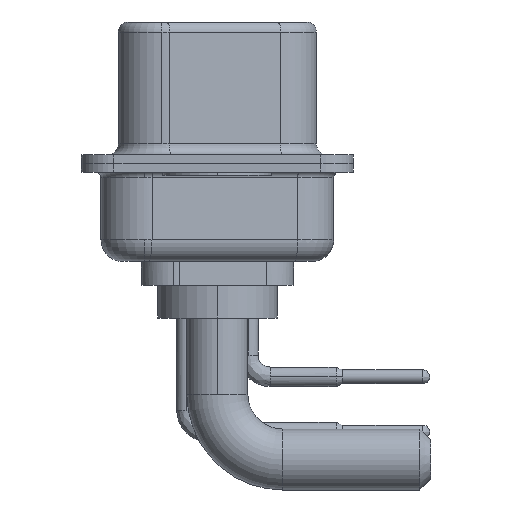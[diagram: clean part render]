
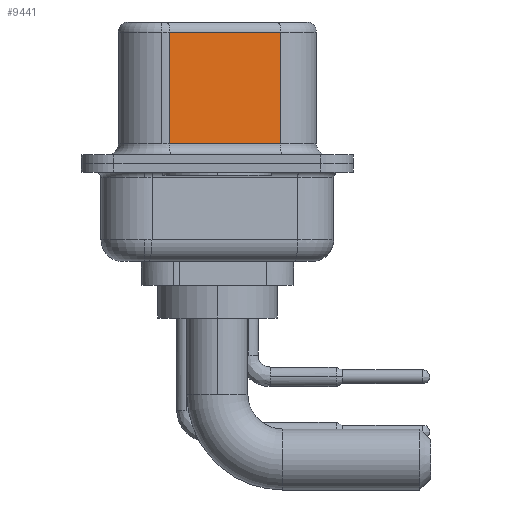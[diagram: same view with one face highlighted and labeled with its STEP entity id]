
A CAD part, left-side view. The second image highlights one B-rep face of the part: STEP entity #9441.
In plain terms, the highlighted planar face has unit normal (-0.985, -0.174, 0).
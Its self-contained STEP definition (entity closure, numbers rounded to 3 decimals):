
#51 = VERTEX_POINT ( 'NONE', #4802 ) ;
#521 = EDGE_CURVE ( 'NONE', #51, #2622, #3120, .T. ) ;
#622 = VECTOR ( 'NONE', #1052, 1000. ) ;
#881 = VECTOR ( 'NONE', #7619, 1000. ) ;
#1052 = DIRECTION ( 'NONE',  ( 0., 0., -1. ) ) ;
#1606 = DIRECTION ( 'NONE',  ( 0., 0., -1. ) ) ;
#1619 = FACE_OUTER_BOUND ( 'NONE', #7997, .T. ) ;
#2414 = CARTESIAN_POINT ( 'NONE',  ( 4.58, -2.897, 0.9 ) ) ;
#2622 = VERTEX_POINT ( 'NONE', #2414 ) ;
#3120 = LINE ( 'NONE', #12028, #15131 ) ;
#4802 = CARTESIAN_POINT ( 'NONE',  ( 3.68, 2.203, 0.9 ) ) ;
#5109 = PLANE ( 'NONE',  #15788 ) ;
#6396 = EDGE_CURVE ( 'NONE', #9933, #2622, #8262, .T. ) ;
#7048 = CARTESIAN_POINT ( 'NONE',  ( 4.58, -2.897, 6.02 ) ) ;
#7619 = DIRECTION ( 'NONE',  ( -0.174, 0.985, 0. ) ) ;
#7997 = EDGE_LOOP ( 'NONE', ( #20481, #19093, #16789, #13719 ) ) ;
#8262 = LINE ( 'NONE', #20416, #622 ) ;
#8454 = CARTESIAN_POINT ( 'NONE',  ( 3.68, 2.203, 6.52 ) ) ;
#8680 = LINE ( 'NONE', #8454, #10190 ) ;
#9441 = ADVANCED_FACE ( 'NONE', ( #1619 ), #5109, .F. ) ;
#9933 = VERTEX_POINT ( 'NONE', #7048 ) ;
#10190 = VECTOR ( 'NONE', #1606, 1000. ) ;
#10282 = DIRECTION ( 'NONE',  ( 0.174, -0.985, 0. ) ) ;
#12028 = CARTESIAN_POINT ( 'NONE',  ( 4.58, -2.897, 0.9 ) ) ;
#12046 = CARTESIAN_POINT ( 'NONE',  ( 4.58, -2.897, 6.52 ) ) ;
#13192 = EDGE_CURVE ( 'NONE', #9933, #13405, #18045, .T. ) ;
#13405 = VERTEX_POINT ( 'NONE', #13735 ) ;
#13719 = ORIENTED_EDGE ( 'NONE', *, *, #521, .T. ) ;
#13735 = CARTESIAN_POINT ( 'NONE',  ( 3.68, 2.203, 6.02 ) ) ;
#13774 = DIRECTION ( 'NONE',  ( -0.174, 0.985, 0. ) ) ;
#14992 = CARTESIAN_POINT ( 'NONE',  ( 4.58, -2.897, 6.02 ) ) ;
#15131 = VECTOR ( 'NONE', #10282, 1000. ) ;
#15740 = EDGE_CURVE ( 'NONE', #13405, #51, #8680, .T. ) ;
#15788 = AXIS2_PLACEMENT_3D ( 'NONE', #12046, #19228, #13774 ) ;
#16789 = ORIENTED_EDGE ( 'NONE', *, *, #15740, .T. ) ;
#18045 = LINE ( 'NONE', #14992, #881 ) ;
#19093 = ORIENTED_EDGE ( 'NONE', *, *, #13192, .T. ) ;
#19228 = DIRECTION ( 'NONE',  ( 0.985, 0.174, 0. ) ) ;
#20416 = CARTESIAN_POINT ( 'NONE',  ( 4.58, -2.897, 6.52 ) ) ;
#20481 = ORIENTED_EDGE ( 'NONE', *, *, #6396, .F. ) ;
